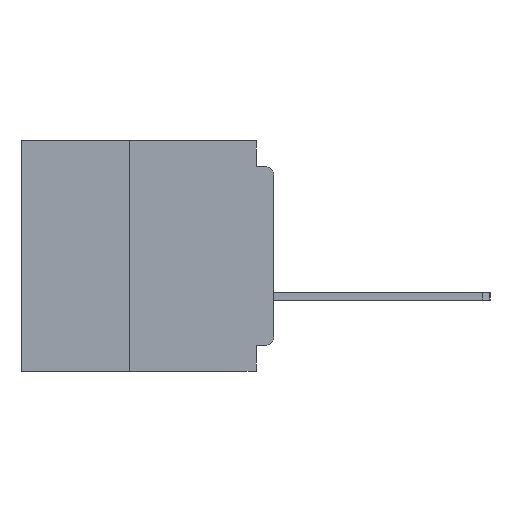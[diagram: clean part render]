
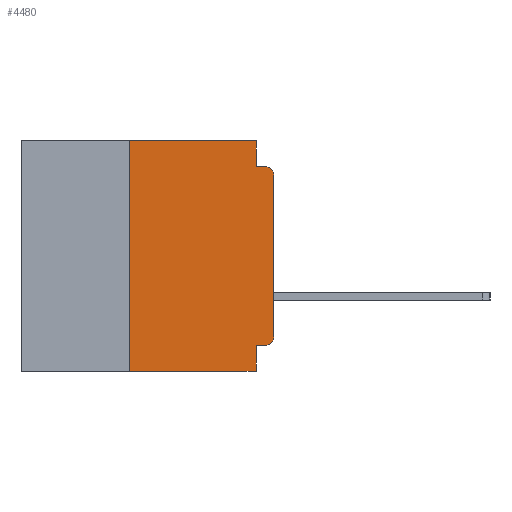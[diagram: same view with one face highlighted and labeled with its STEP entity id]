
A CAD part, left-side view. The second image highlights one B-rep face of the part: STEP entity #4480.
In plain terms, the highlighted planar face has unit normal (-1, 0, 0).
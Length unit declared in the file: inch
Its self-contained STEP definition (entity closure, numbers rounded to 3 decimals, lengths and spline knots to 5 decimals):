
#2224 = DIRECTION ( 'NONE',  ( 0., -1., 0. ) ) ;
#4278 = ORIENTED_EDGE ( 'NONE', *, *, #35151, .T. ) ;
#4327 = CARTESIAN_POINT ( 'NONE',  ( 0., 0., -0.34 ) ) ;
#4405 = VERTEX_POINT ( 'NONE', #4327 ) ;
#4480 = ADVANCED_FACE ( 'NONE', ( #23620 ), #4733, .F. ) ;
#4666 = VECTOR ( 'NONE', #9038, 39.37008 ) ;
#4733 = PLANE ( 'NONE',  #36562 ) ;
#5998 = ORIENTED_EDGE ( 'NONE', *, *, #49039, .T. ) ;
#6420 = EDGE_CURVE ( 'NONE', #15071, #26982, #55417, .T. ) ;
#6468 = VECTOR ( 'NONE', #12011, 39.37008 ) ;
#6930 = CARTESIAN_POINT ( 'NONE',  ( 0., 0., 0. ) ) ;
#6960 = CARTESIAN_POINT ( 'NONE',  ( 0., 0.25, -0.4 ) ) ;
#7184 = EDGE_CURVE ( 'NONE', #22876, #15071, #53246, .T. ) ;
#7497 = CARTESIAN_POINT ( 'NONE',  ( 0., 0.031, -0.4 ) ) ;
#7935 = LINE ( 'NONE', #30246, #6468 ) ;
#8321 = VERTEX_POINT ( 'NONE', #49764 ) ;
#8737 = VERTEX_POINT ( 'NONE', #6960 ) ;
#9038 = DIRECTION ( 'NONE',  ( 0., 1., 0. ) ) ;
#9212 = VERTEX_POINT ( 'NONE', #29113 ) ;
#9540 = LINE ( 'NONE', #13522, #32469 ) ;
#10457 = DIRECTION ( 'NONE',  ( -1., 0., 0. ) ) ;
#10790 = DIRECTION ( 'NONE',  ( -1., 0., 0. ) ) ;
#11653 = CARTESIAN_POINT ( 'NONE',  ( 0., 0.031, -0.045 ) ) ;
#12011 = DIRECTION ( 'NONE',  ( 0., -1., 0. ) ) ;
#12148 = ORIENTED_EDGE ( 'NONE', *, *, #21146, .F. ) ;
#12602 = AXIS2_PLACEMENT_3D ( 'NONE', #37861, #10457, #42451 ) ;
#13522 = CARTESIAN_POINT ( 'NONE',  ( 0., 0.031, 0. ) ) ;
#13724 = DIRECTION ( 'NONE',  ( 0., 0., -1. ) ) ;
#13959 = CARTESIAN_POINT ( 'NONE',  ( 0., 0.437, 0. ) ) ;
#14305 = EDGE_LOOP ( 'NONE', ( #5998, #4278, #26586, #21063, #27383, #12148, #46976, #37714, #20485, #35166 ) ) ;
#14750 = LINE ( 'NONE', #19122, #25538 ) ;
#15071 = VERTEX_POINT ( 'NONE', #22981 ) ;
#17156 = EDGE_CURVE ( 'NONE', #8321, #9212, #25344, .T. ) ;
#17783 = LINE ( 'NONE', #6930, #52666 ) ;
#18301 = CARTESIAN_POINT ( 'NONE',  ( 0., 0., -0.355 ) ) ;
#18327 = CIRCLE ( 'NONE', #12602, 0.015 ) ;
#18441 = VERTEX_POINT ( 'NONE', #43172 ) ;
#18619 = DIRECTION ( 'NONE',  ( 0., 0., -1. ) ) ;
#19122 = CARTESIAN_POINT ( 'NONE',  ( 0., 0.437, -0.4 ) ) ;
#19907 = LINE ( 'NONE', #31673, #42723 ) ;
#20485 = ORIENTED_EDGE ( 'NONE', *, *, #7184, .F. ) ;
#20924 = VERTEX_POINT ( 'NONE', #11653 ) ;
#21063 = ORIENTED_EDGE ( 'NONE', *, *, #43340, .F. ) ;
#21146 = EDGE_CURVE ( 'NONE', #8737, #8321, #19907, .T. ) ;
#22876 = VERTEX_POINT ( 'NONE', #36428 ) ;
#22981 = CARTESIAN_POINT ( 'NONE',  ( 0., 0.031, -0.355 ) ) ;
#23620 = FACE_OUTER_BOUND ( 'NONE', #14305, .T. ) ;
#25344 = LINE ( 'NONE', #56974, #50955 ) ;
#25538 = VECTOR ( 'NONE', #50969, 39.37008 ) ;
#26586 = ORIENTED_EDGE ( 'NONE', *, *, #38025, .F. ) ;
#26716 = CARTESIAN_POINT ( 'NONE',  ( 0., 0.031, -0.4 ) ) ;
#26982 = VERTEX_POINT ( 'NONE', #26716 ) ;
#27383 = ORIENTED_EDGE ( 'NONE', *, *, #17156, .F. ) ;
#29113 = CARTESIAN_POINT ( 'NONE',  ( 0., 0.031, 0. ) ) ;
#30246 = CARTESIAN_POINT ( 'NONE',  ( 0., 0., -0.045 ) ) ;
#31673 = CARTESIAN_POINT ( 'NONE',  ( 0., 0.25, -0.4 ) ) ;
#32469 = VECTOR ( 'NONE', #13724, 39.37008 ) ;
#35151 = EDGE_CURVE ( 'NONE', #38215, #18441, #18327, .T. ) ;
#35166 = ORIENTED_EDGE ( 'NONE', *, *, #44206, .T. ) ;
#36428 = CARTESIAN_POINT ( 'NONE',  ( 0., 0.015, -0.355 ) ) ;
#36562 = AXIS2_PLACEMENT_3D ( 'NONE', #13959, #45901, #18619 ) ;
#37714 = ORIENTED_EDGE ( 'NONE', *, *, #6420, .F. ) ;
#37861 = CARTESIAN_POINT ( 'NONE',  ( 0., 0.015, -0.06 ) ) ;
#38025 = EDGE_CURVE ( 'NONE', #20924, #18441, #7935, .T. ) ;
#38183 = CARTESIAN_POINT ( 'NONE',  ( 0., 0.015, -0.34 ) ) ;
#38215 = VERTEX_POINT ( 'NONE', #40794 ) ;
#38744 = DIRECTION ( 'NONE',  ( 0., 0., 1. ) ) ;
#40794 = CARTESIAN_POINT ( 'NONE',  ( 0., 0., -0.06 ) ) ;
#42451 = DIRECTION ( 'NONE',  ( 0., 0., -1. ) ) ;
#42723 = VECTOR ( 'NONE', #49791, 39.37008 ) ;
#42789 = DIRECTION ( 'NONE',  ( 0., 0., -1. ) ) ;
#43172 = CARTESIAN_POINT ( 'NONE',  ( 0., 0.015, -0.045 ) ) ;
#43340 = EDGE_CURVE ( 'NONE', #9212, #20924, #9540, .T. ) ;
#43398 = VECTOR ( 'NONE', #52990, 39.37008 ) ;
#44206 = EDGE_CURVE ( 'NONE', #22876, #4405, #45897, .T. ) ;
#45897 = CIRCLE ( 'NONE', #56895, 0.015 ) ;
#45901 = DIRECTION ( 'NONE',  ( 1., 0., 0. ) ) ;
#46976 = ORIENTED_EDGE ( 'NONE', *, *, #49935, .T. ) ;
#49039 = EDGE_CURVE ( 'NONE', #4405, #38215, #17783, .T. ) ;
#49764 = CARTESIAN_POINT ( 'NONE',  ( 0., 0.25, 0. ) ) ;
#49791 = DIRECTION ( 'NONE',  ( 0., 0., 1. ) ) ;
#49935 = EDGE_CURVE ( 'NONE', #8737, #26982, #14750, .T. ) ;
#50955 = VECTOR ( 'NONE', #2224, 39.37008 ) ;
#50969 = DIRECTION ( 'NONE',  ( 0., -1., 0. ) ) ;
#52666 = VECTOR ( 'NONE', #38744, 39.37008 ) ;
#52990 = DIRECTION ( 'NONE',  ( 0., 0., -1. ) ) ;
#53246 = LINE ( 'NONE', #18301, #4666 ) ;
#55417 = LINE ( 'NONE', #7497, #43398 ) ;
#56895 = AXIS2_PLACEMENT_3D ( 'NONE', #38183, #10790, #42789 ) ;
#56974 = CARTESIAN_POINT ( 'NONE',  ( 0., 0.437, 0. ) ) ;
